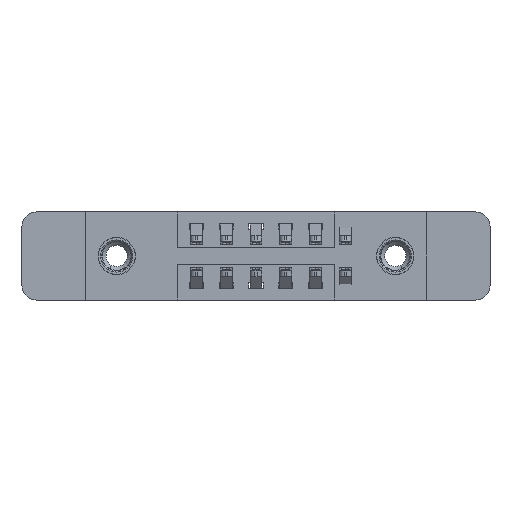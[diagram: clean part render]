
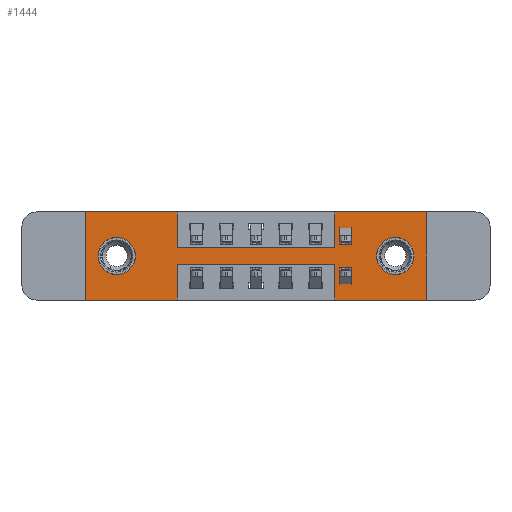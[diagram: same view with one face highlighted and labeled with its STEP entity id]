
A CAD part, front view. The second image highlights one B-rep face of the part: STEP entity #1444.
In plain terms, the highlighted planar face has unit normal (0, -1, 0).
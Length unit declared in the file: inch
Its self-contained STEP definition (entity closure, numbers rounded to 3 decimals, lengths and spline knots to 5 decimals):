
#27 = CARTESIAN_POINT ( 'NONE',  ( 1.0475, 0., 0. ) ) ;
#116 = EDGE_CURVE ( 'NONE', #10281, #8883, #11533, .T. ) ;
#190 = VECTOR ( 'NONE', #8134, 39.37008 ) ;
#236 = ORIENTED_EDGE ( 'NONE', *, *, #937, .T. ) ;
#524 = AXIS2_PLACEMENT_3D ( 'NONE', #2425, #8207, #6833 ) ;
#579 = DIRECTION ( 'NONE',  ( 0., 0., -1. ) ) ;
#613 = DIRECTION ( 'NONE',  ( 0., 0., -1. ) ) ;
#697 = VERTEX_POINT ( 'NONE', #2306 ) ;
#937 = EDGE_CURVE ( 'NONE', #2758, #2372, #2156, .T. ) ;
#1241 = CARTESIAN_POINT ( 'NONE',  ( 0., 0., -0.37 ) ) ;
#1252 = FACE_BOUND ( 'NONE', #5935, .T. ) ;
#1289 = VECTOR ( 'NONE', #4406, 39.37008 ) ;
#1329 = VERTEX_POINT ( 'NONE', #9623 ) ;
#1444 = ADVANCED_FACE ( 'NONE', ( #1550, #1252, #10325 ), #3582, .T. ) ;
#1530 = ORIENTED_EDGE ( 'NONE', *, *, #10661, .T. ) ;
#1550 = FACE_BOUND ( 'NONE', #2126, .T. ) ;
#1764 = AXIS2_PLACEMENT_3D ( 'NONE', #10309, #7988, #5870 ) ;
#1820 = CARTESIAN_POINT ( 'NONE',  ( 1.0475, 0., -0.37 ) ) ;
#1878 = ORIENTED_EDGE ( 'NONE', *, *, #3613, .F. ) ;
#1926 = CARTESIAN_POINT ( 'NONE',  ( 0.1325, 0., -0.185 ) ) ;
#2060 = VECTOR ( 'NONE', #13106, 39.37008 ) ;
#2126 = EDGE_LOOP ( 'NONE', ( #236, #1530 ) ) ;
#2156 = CIRCLE ( 'NONE', #10206, 0.078 ) ;
#2306 = CARTESIAN_POINT ( 'NONE',  ( 1.0475, 0., -0.15 ) ) ;
#2333 = VERTEX_POINT ( 'NONE', #4287 ) ;
#2372 = VERTEX_POINT ( 'NONE', #3010 ) ;
#2425 = CARTESIAN_POINT ( 'NONE',  ( 0., 0., -0.37 ) ) ;
#2603 = CARTESIAN_POINT ( 'NONE',  ( 0., 0., 0. ) ) ;
#2694 = CARTESIAN_POINT ( 'NONE',  ( 1.435, 0., -0.37 ) ) ;
#2758 = VERTEX_POINT ( 'NONE', #3050 ) ;
#2760 = VERTEX_POINT ( 'NONE', #12276 ) ;
#2775 = VERTEX_POINT ( 'NONE', #12368 ) ;
#2959 = EDGE_CURVE ( 'NONE', #2775, #10281, #6069, .T. ) ;
#2986 = EDGE_CURVE ( 'NONE', #5854, #2333, #8944, .T. ) ;
#3010 = CARTESIAN_POINT ( 'NONE',  ( 1.3025, 0., -0.263 ) ) ;
#3050 = CARTESIAN_POINT ( 'NONE',  ( 1.3025, 0., -0.107 ) ) ;
#3161 = CARTESIAN_POINT ( 'NONE',  ( 0.1325, 0., -0.185 ) ) ;
#3233 = ORIENTED_EDGE ( 'NONE', *, *, #7047, .T. ) ;
#3272 = CIRCLE ( 'NONE', #5615, 0.078 ) ;
#3391 = CARTESIAN_POINT ( 'NONE',  ( 0.1325, 0., -0.263 ) ) ;
#3430 = ORIENTED_EDGE ( 'NONE', *, *, #11167, .F. ) ;
#3436 = CARTESIAN_POINT ( 'NONE',  ( 1.0475, 0., -0.22 ) ) ;
#3582 = PLANE ( 'NONE',  #524 ) ;
#3613 = EDGE_CURVE ( 'NONE', #11380, #3828, #5048, .T. ) ;
#3808 = ORIENTED_EDGE ( 'NONE', *, *, #4912, .F. ) ;
#3828 = VERTEX_POINT ( 'NONE', #2694 ) ;
#4089 = DIRECTION ( 'NONE',  ( 0., 0., 1. ) ) ;
#4174 = ORIENTED_EDGE ( 'NONE', *, *, #2986, .F. ) ;
#4287 = CARTESIAN_POINT ( 'NONE',  ( 0.3875, 0., -0.37 ) ) ;
#4406 = DIRECTION ( 'NONE',  ( 0., 0., 1. ) ) ;
#4434 = DIRECTION ( 'NONE',  ( 1., 0., 0. ) ) ;
#4617 = ORIENTED_EDGE ( 'NONE', *, *, #8035, .F. ) ;
#4761 = EDGE_CURVE ( 'NONE', #3828, #11937, #11963, .T. ) ;
#4823 = EDGE_CURVE ( 'NONE', #2760, #11380, #5523, .T. ) ;
#4912 = EDGE_CURVE ( 'NONE', #2333, #7719, #9187, .T. ) ;
#4921 = ORIENTED_EDGE ( 'NONE', *, *, #13531, .F. ) ;
#5048 = LINE ( 'NONE', #9507, #9799 ) ;
#5106 = DIRECTION ( 'NONE',  ( 0., 1., 0. ) ) ;
#5298 = VECTOR ( 'NONE', #4434, 39.37008 ) ;
#5523 = LINE ( 'NONE', #12120, #5298 ) ;
#5615 = AXIS2_PLACEMENT_3D ( 'NONE', #1926, #6346, #8309 ) ;
#5675 = CIRCLE ( 'NONE', #13683, 0.078 ) ;
#5728 = VECTOR ( 'NONE', #12623, 39.37008 ) ;
#5854 = VERTEX_POINT ( 'NONE', #13796 ) ;
#5870 = DIRECTION ( 'NONE',  ( 0., 0., -1. ) ) ;
#5888 = CARTESIAN_POINT ( 'NONE',  ( 0.3875, 0., 0. ) ) ;
#5935 = EDGE_LOOP ( 'NONE', ( #9864, #3233 ) ) ;
#6022 = ORIENTED_EDGE ( 'NONE', *, *, #4823, .F. ) ;
#6069 = LINE ( 'NONE', #2603, #8213 ) ;
#6346 = DIRECTION ( 'NONE',  ( 0., 1., 0. ) ) ;
#6349 = DIRECTION ( 'NONE',  ( 1., 0., 0. ) ) ;
#6409 = DIRECTION ( 'NONE',  ( 0., 0., 1. ) ) ;
#6477 = CARTESIAN_POINT ( 'NONE',  ( 0., 0., 0. ) ) ;
#6586 = CIRCLE ( 'NONE', #1764, 0.078 ) ;
#6627 = CARTESIAN_POINT ( 'NONE',  ( 1.435, 0., 0. ) ) ;
#6641 = DIRECTION ( 'NONE',  ( 0., 0., -1. ) ) ;
#6725 = CARTESIAN_POINT ( 'NONE',  ( 0., 0., -0.37 ) ) ;
#6758 = VECTOR ( 'NONE', #8646, 39.37008 ) ;
#6833 = DIRECTION ( 'NONE',  ( 0., 0., -1. ) ) ;
#7047 = EDGE_CURVE ( 'NONE', #8096, #1329, #3272, .T. ) ;
#7719 = VERTEX_POINT ( 'NONE', #6725 ) ;
#7988 = DIRECTION ( 'NONE',  ( 0., 1., 0. ) ) ;
#8035 = EDGE_CURVE ( 'NONE', #12089, #5854, #14069, .T. ) ;
#8059 = DIRECTION ( 'NONE',  ( 0., 1., 0. ) ) ;
#8096 = VERTEX_POINT ( 'NONE', #3391 ) ;
#8134 = DIRECTION ( 'NONE',  ( -1., 0., 0. ) ) ;
#8201 = CARTESIAN_POINT ( 'NONE',  ( 0., 0., -0.37 ) ) ;
#8207 = DIRECTION ( 'NONE',  ( 0., -1., 0. ) ) ;
#8213 = VECTOR ( 'NONE', #10218, 39.37008 ) ;
#8309 = DIRECTION ( 'NONE',  ( 0., 0., 1. ) ) ;
#8508 = CARTESIAN_POINT ( 'NONE',  ( 0.3875, 0., -0.22 ) ) ;
#8646 = DIRECTION ( 'NONE',  ( -1., 0., 0. ) ) ;
#8658 = VECTOR ( 'NONE', #6641, 39.37008 ) ;
#8883 = VERTEX_POINT ( 'NONE', #13953 ) ;
#8944 = LINE ( 'NONE', #12218, #8658 ) ;
#9044 = DIRECTION ( 'NONE',  ( 0., 0., -1. ) ) ;
#9187 = LINE ( 'NONE', #8201, #190 ) ;
#9204 = EDGE_CURVE ( 'NONE', #697, #2760, #12161, .T. ) ;
#9340 = VECTOR ( 'NONE', #4089, 39.37008 ) ;
#9486 = LINE ( 'NONE', #6477, #9340 ) ;
#9496 = EDGE_CURVE ( 'NONE', #8883, #697, #11843, .T. ) ;
#9507 = CARTESIAN_POINT ( 'NONE',  ( 1.435, 0., 0. ) ) ;
#9623 = CARTESIAN_POINT ( 'NONE',  ( 0.1325, 0., -0.107 ) ) ;
#9632 = CARTESIAN_POINT ( 'NONE',  ( 0.3875, 0., -0.15 ) ) ;
#9799 = VECTOR ( 'NONE', #613, 39.37008 ) ;
#9864 = ORIENTED_EDGE ( 'NONE', *, *, #11151, .T. ) ;
#10206 = AXIS2_PLACEMENT_3D ( 'NONE', #10307, #8059, #9044 ) ;
#10218 = DIRECTION ( 'NONE',  ( 1., 0., 0. ) ) ;
#10281 = VERTEX_POINT ( 'NONE', #5888 ) ;
#10307 = CARTESIAN_POINT ( 'NONE',  ( 1.3025, 0., -0.185 ) ) ;
#10309 = CARTESIAN_POINT ( 'NONE',  ( 1.3025, 0., -0.185 ) ) ;
#10325 = FACE_OUTER_BOUND ( 'NONE', #13661, .T. ) ;
#10394 = ORIENTED_EDGE ( 'NONE', *, *, #116, .F. ) ;
#10457 = CARTESIAN_POINT ( 'NONE',  ( 0.3875, 0., 0. ) ) ;
#10661 = EDGE_CURVE ( 'NONE', #2372, #2758, #6586, .T. ) ;
#11151 = EDGE_CURVE ( 'NONE', #1329, #8096, #5675, .T. ) ;
#11167 = EDGE_CURVE ( 'NONE', #7719, #2775, #9486, .T. ) ;
#11290 = ORIENTED_EDGE ( 'NONE', *, *, #2959, .F. ) ;
#11371 = ORIENTED_EDGE ( 'NONE', *, *, #9496, .F. ) ;
#11380 = VERTEX_POINT ( 'NONE', #6627 ) ;
#11533 = LINE ( 'NONE', #10457, #13846 ) ;
#11790 = ORIENTED_EDGE ( 'NONE', *, *, #9204, .F. ) ;
#11843 = LINE ( 'NONE', #9632, #12999 ) ;
#11920 = ORIENTED_EDGE ( 'NONE', *, *, #4761, .F. ) ;
#11937 = VERTEX_POINT ( 'NONE', #14117 ) ;
#11963 = LINE ( 'NONE', #1241, #2060 ) ;
#12089 = VERTEX_POINT ( 'NONE', #3436 ) ;
#12120 = CARTESIAN_POINT ( 'NONE',  ( 0., 0., 0. ) ) ;
#12161 = LINE ( 'NONE', #27, #1289 ) ;
#12218 = CARTESIAN_POINT ( 'NONE',  ( 0.3875, 0., -0.37 ) ) ;
#12276 = CARTESIAN_POINT ( 'NONE',  ( 1.0475, 0., 0. ) ) ;
#12368 = CARTESIAN_POINT ( 'NONE',  ( 0., 0., 0. ) ) ;
#12623 = DIRECTION ( 'NONE',  ( 0., 0., 1. ) ) ;
#12749 = LINE ( 'NONE', #1820, #5728 ) ;
#12999 = VECTOR ( 'NONE', #6349, 39.37008 ) ;
#13106 = DIRECTION ( 'NONE',  ( -1., 0., 0. ) ) ;
#13531 = EDGE_CURVE ( 'NONE', #11937, #12089, #12749, .T. ) ;
#13661 = EDGE_LOOP ( 'NONE', ( #4174, #4617, #4921, #11920, #1878, #6022, #11790, #11371, #10394, #11290, #3430, #3808 ) ) ;
#13683 = AXIS2_PLACEMENT_3D ( 'NONE', #3161, #5106, #6409 ) ;
#13796 = CARTESIAN_POINT ( 'NONE',  ( 0.3875, 0., -0.22 ) ) ;
#13846 = VECTOR ( 'NONE', #579, 39.37008 ) ;
#13953 = CARTESIAN_POINT ( 'NONE',  ( 0.3875, 0., -0.15 ) ) ;
#14069 = LINE ( 'NONE', #8508, #6758 ) ;
#14117 = CARTESIAN_POINT ( 'NONE',  ( 1.0475, 0., -0.37 ) ) ;
